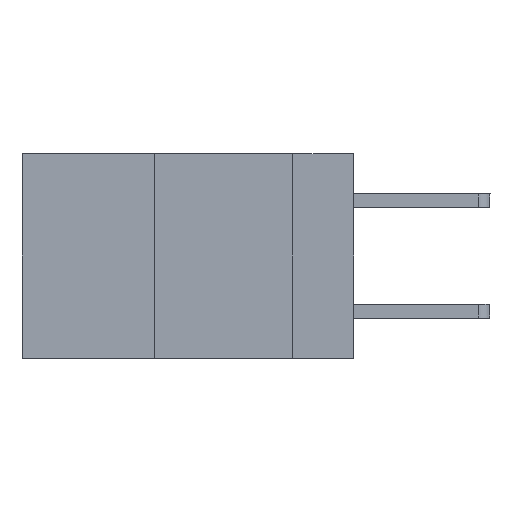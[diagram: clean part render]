
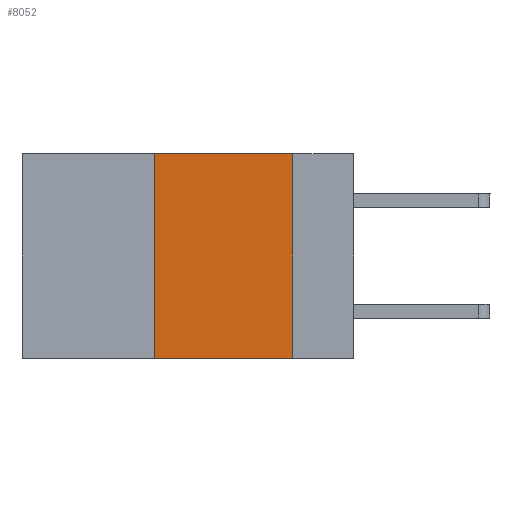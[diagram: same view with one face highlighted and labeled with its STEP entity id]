
A CAD part, left-side view. The second image highlights one B-rep face of the part: STEP entity #8052.
In plain terms, the highlighted planar face has unit normal (-1, 0, 0).
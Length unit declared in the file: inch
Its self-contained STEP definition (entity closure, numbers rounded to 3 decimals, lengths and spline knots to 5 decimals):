
#306 = CARTESIAN_POINT ( 'NONE',  ( 0., 0.36, 0. ) ) ;
#1015 = AXIS2_PLACEMENT_3D ( 'NONE', #1255, #4547, #3043 ) ;
#1221 = LINE ( 'NONE', #306, #1837 ) ;
#1255 = CARTESIAN_POINT ( 'NONE',  ( 0., 0.6, 0. ) ) ;
#1837 = VECTOR ( 'NONE', #3596, 39.37008 ) ;
#1906 = DIRECTION ( 'NONE',  ( 0., 0., -1. ) ) ;
#2068 = FACE_OUTER_BOUND ( 'NONE', #5324, .T. ) ;
#2231 = PLANE ( 'NONE',  #1015 ) ;
#2296 = CARTESIAN_POINT ( 'NONE',  ( 0., 0.36, -0.37 ) ) ;
#2529 = DIRECTION ( 'NONE',  ( 0., -1., 0. ) ) ;
#3043 = DIRECTION ( 'NONE',  ( 0., 0., -1. ) ) ;
#3124 = CARTESIAN_POINT ( 'NONE',  ( 0., 0.11, 0. ) ) ;
#3231 = VERTEX_POINT ( 'NONE', #8849 ) ;
#3241 = CARTESIAN_POINT ( 'NONE',  ( 0., 0.6, -0.37 ) ) ;
#3392 = LINE ( 'NONE', #3241, #4600 ) ;
#3596 = DIRECTION ( 'NONE',  ( 0., 0., 1. ) ) ;
#3949 = CARTESIAN_POINT ( 'NONE',  ( 0., 0.6, 0. ) ) ;
#4256 = EDGE_CURVE ( 'NONE', #7565, #3231, #1221, .T. ) ;
#4283 = CARTESIAN_POINT ( 'NONE',  ( 0., 0.11, 0. ) ) ;
#4547 = DIRECTION ( 'NONE',  ( 1., 0., 0. ) ) ;
#4600 = VECTOR ( 'NONE', #2529, 39.37008 ) ;
#4745 = LINE ( 'NONE', #3949, #8947 ) ;
#5324 = EDGE_LOOP ( 'NONE', ( #9197, #9833, #6638, #9889 ) ) ;
#5472 = EDGE_CURVE ( 'NONE', #7565, #7014, #3392, .T. ) ;
#5918 = VERTEX_POINT ( 'NONE', #3124 ) ;
#6546 = EDGE_CURVE ( 'NONE', #5918, #7014, #7751, .T. ) ;
#6638 = ORIENTED_EDGE ( 'NONE', *, *, #4256, .F. ) ;
#7014 = VERTEX_POINT ( 'NONE', #8397 ) ;
#7255 = DIRECTION ( 'NONE',  ( 0., -1., 0. ) ) ;
#7298 = EDGE_CURVE ( 'NONE', #3231, #5918, #4745, .T. ) ;
#7565 = VERTEX_POINT ( 'NONE', #2296 ) ;
#7751 = LINE ( 'NONE', #4283, #10298 ) ;
#8052 = ADVANCED_FACE ( 'NONE', ( #2068 ), #2231, .F. ) ;
#8397 = CARTESIAN_POINT ( 'NONE',  ( 0., 0.11, -0.37 ) ) ;
#8849 = CARTESIAN_POINT ( 'NONE',  ( 0., 0.36, 0. ) ) ;
#8947 = VECTOR ( 'NONE', #7255, 39.37008 ) ;
#9197 = ORIENTED_EDGE ( 'NONE', *, *, #6546, .F. ) ;
#9833 = ORIENTED_EDGE ( 'NONE', *, *, #7298, .F. ) ;
#9889 = ORIENTED_EDGE ( 'NONE', *, *, #5472, .T. ) ;
#10298 = VECTOR ( 'NONE', #1906, 39.37008 ) ;
